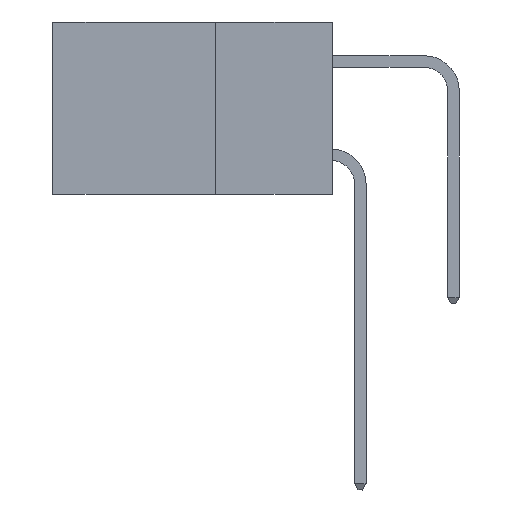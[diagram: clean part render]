
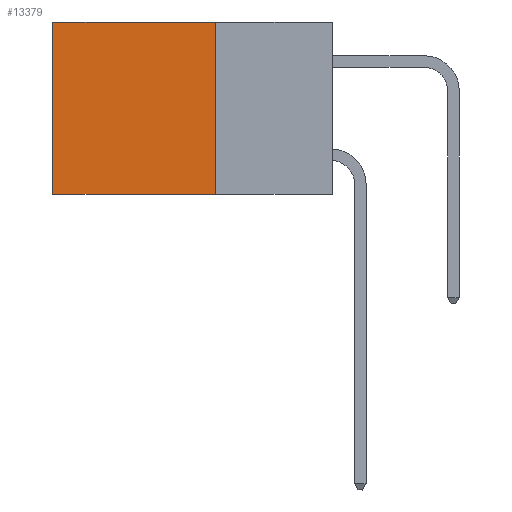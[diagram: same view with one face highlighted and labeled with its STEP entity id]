
A CAD part, left-side view. The second image highlights one B-rep face of the part: STEP entity #13379.
In plain terms, the highlighted planar face has unit normal (-1, 0, 0).
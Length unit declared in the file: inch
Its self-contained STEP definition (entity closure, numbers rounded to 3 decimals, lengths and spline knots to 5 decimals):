
#488 = EDGE_CURVE ( 'NONE', #10683, #11335, #4000, .T. ) ;
#579 = VECTOR ( 'NONE', #4859, 39.37008 ) ;
#723 = FACE_OUTER_BOUND ( 'NONE', #817, .T. ) ;
#817 = EDGE_LOOP ( 'NONE', ( #2359, #2907, #6969, #5380 ) ) ;
#1539 = DIRECTION ( 'NONE',  ( 1., 0., 0. ) ) ;
#1597 = VECTOR ( 'NONE', #12785, 39.37008 ) ;
#2098 = CARTESIAN_POINT ( 'NONE',  ( 0.2615, 0.6, 0. ) ) ;
#2359 = ORIENTED_EDGE ( 'NONE', *, *, #10025, .T. ) ;
#2679 = DIRECTION ( 'NONE',  ( 0., 0., -1. ) ) ;
#2890 = DIRECTION ( 'NONE',  ( 0., 0., -1. ) ) ;
#2907 = ORIENTED_EDGE ( 'NONE', *, *, #12526, .F. ) ;
#3565 = CARTESIAN_POINT ( 'NONE',  ( 0.2615, 0.25, 0. ) ) ;
#3737 = DIRECTION ( 'NONE',  ( 0., 1., 0. ) ) ;
#4000 = LINE ( 'NONE', #5979, #13165 ) ;
#4376 = CARTESIAN_POINT ( 'NONE',  ( 0.2615, 0.6, -0.37 ) ) ;
#4577 = LINE ( 'NONE', #8566, #1597 ) ;
#4859 = DIRECTION ( 'NONE',  ( 0., 1., 0. ) ) ;
#5380 = ORIENTED_EDGE ( 'NONE', *, *, #5420, .T. ) ;
#5420 = EDGE_CURVE ( 'NONE', #10683, #8544, #11133, .T. ) ;
#5454 = VECTOR ( 'NONE', #3737, 39.37008 ) ;
#5979 = CARTESIAN_POINT ( 'NONE',  ( 0.2615, 0.25, -0.37 ) ) ;
#6969 = ORIENTED_EDGE ( 'NONE', *, *, #488, .F. ) ;
#7031 = VERTEX_POINT ( 'NONE', #4376 ) ;
#8544 = VERTEX_POINT ( 'NONE', #2098 ) ;
#8566 = CARTESIAN_POINT ( 'NONE',  ( 0.2615, 0.6, -0.37 ) ) ;
#9006 = PLANE ( 'NONE',  #12450 ) ;
#9365 = CARTESIAN_POINT ( 'NONE',  ( 0.2615, 0.25, -0.37 ) ) ;
#10025 = EDGE_CURVE ( 'NONE', #8544, #7031, #4577, .T. ) ;
#10270 = LINE ( 'NONE', #11230, #579 ) ;
#10683 = VERTEX_POINT ( 'NONE', #3565 ) ;
#11133 = LINE ( 'NONE', #11200, #5454 ) ;
#11200 = CARTESIAN_POINT ( 'NONE',  ( 0.2615, 0.25, 0. ) ) ;
#11230 = CARTESIAN_POINT ( 'NONE',  ( 0.2615, 0.25, -0.37 ) ) ;
#11335 = VERTEX_POINT ( 'NONE', #9365 ) ;
#11989 = CARTESIAN_POINT ( 'NONE',  ( 0.2615, 0.25, -0.37 ) ) ;
#12450 = AXIS2_PLACEMENT_3D ( 'NONE', #11989, #1539, #2679 ) ;
#12526 = EDGE_CURVE ( 'NONE', #11335, #7031, #10270, .T. ) ;
#12785 = DIRECTION ( 'NONE',  ( 0., 0., -1. ) ) ;
#13165 = VECTOR ( 'NONE', #2890, 39.37008 ) ;
#13379 = ADVANCED_FACE ( 'NONE', ( #723 ), #9006, .F. ) ;
